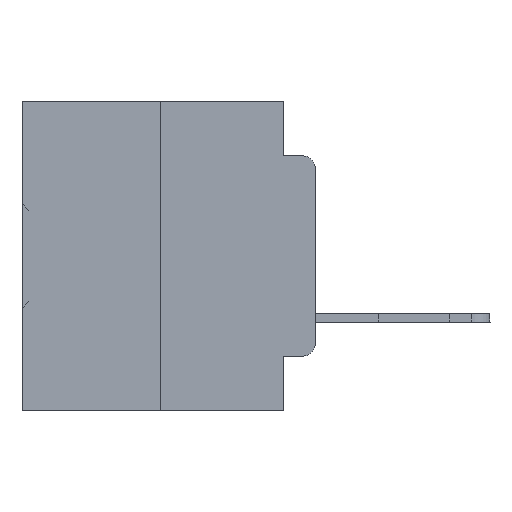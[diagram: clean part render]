
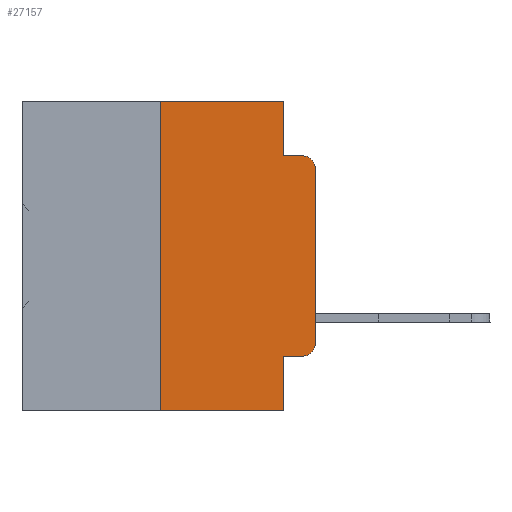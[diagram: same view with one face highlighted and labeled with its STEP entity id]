
A CAD part, left-side view. The second image highlights one B-rep face of the part: STEP entity #27157.
In plain terms, the highlighted planar face has unit normal (-1, 0, 0).
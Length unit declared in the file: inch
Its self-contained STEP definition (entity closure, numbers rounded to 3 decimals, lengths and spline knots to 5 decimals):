
#327 = CARTESIAN_POINT ( 'NONE',  ( 0., 0.25, 0. ) ) ;
#1397 = LINE ( 'NONE', #5929, #7560 ) ;
#1863 = DIRECTION ( 'NONE',  ( 0., -1., 0. ) ) ;
#1883 = CARTESIAN_POINT ( 'NONE',  ( 0., 0.473, 0. ) ) ;
#2228 = DIRECTION ( 'NONE',  ( 0., -1., 0. ) ) ;
#2650 = ORIENTED_EDGE ( 'NONE', *, *, #11590, .T. ) ;
#3807 = CARTESIAN_POINT ( 'NONE',  ( 0., 0., -0.3915 ) ) ;
#3957 = DIRECTION ( 'NONE',  ( 1., 0., 0. ) ) ;
#4090 = EDGE_CURVE ( 'NONE', #22482, #36024, #15081, .T. ) ;
#4218 = DIRECTION ( 'NONE',  ( 0., 0., -1. ) ) ;
#5114 = VECTOR ( 'NONE', #1863, 39.37008 ) ;
#5192 = VECTOR ( 'NONE', #32256, 39.37008 ) ;
#5536 = AXIS2_PLACEMENT_3D ( 'NONE', #11875, #25906, #23444 ) ;
#5929 = CARTESIAN_POINT ( 'NONE',  ( 0., 0.051, 0. ) ) ;
#6291 = LINE ( 'NONE', #33687, #19671 ) ;
#6921 = AXIS2_PLACEMENT_3D ( 'NONE', #27531, #30012, #10509 ) ;
#6992 = ORIENTED_EDGE ( 'NONE', *, *, #33850, .F. ) ;
#7041 = VERTEX_POINT ( 'NONE', #29921 ) ;
#7425 = LINE ( 'NONE', #18552, #5192 ) ;
#7560 = VECTOR ( 'NONE', #31439, 39.37008 ) ;
#8811 = ORIENTED_EDGE ( 'NONE', *, *, #26249, .F. ) ;
#8902 = ORIENTED_EDGE ( 'NONE', *, *, #4090, .T. ) ;
#8966 = AXIS2_PLACEMENT_3D ( 'NONE', #15193, #3957, #4218 ) ;
#9478 = PLANE ( 'NONE',  #8966 ) ;
#10082 = VERTEX_POINT ( 'NONE', #29663 ) ;
#10411 = VERTEX_POINT ( 'NONE', #3807 ) ;
#10509 = DIRECTION ( 'NONE',  ( 0., 0., -1. ) ) ;
#11061 = ORIENTED_EDGE ( 'NONE', *, *, #14763, .T. ) ;
#11104 = CARTESIAN_POINT ( 'NONE',  ( 0., 0.051, -0.0885 ) ) ;
#11590 = EDGE_CURVE ( 'NONE', #36024, #10411, #19796, .T. ) ;
#11759 = CARTESIAN_POINT ( 'NONE',  ( 0., 0.02, -0.4115 ) ) ;
#11875 = CARTESIAN_POINT ( 'NONE',  ( 0., 0.02, -0.1085 ) ) ;
#11906 = VERTEX_POINT ( 'NONE', #15440 ) ;
#12588 = CARTESIAN_POINT ( 'NONE',  ( 0., 0.25, -0.5 ) ) ;
#13746 = ORIENTED_EDGE ( 'NONE', *, *, #13870, .T. ) ;
#13870 = EDGE_CURVE ( 'NONE', #10411, #7041, #6291, .T. ) ;
#14763 = EDGE_CURVE ( 'NONE', #24092, #11906, #30805, .T. ) ;
#15081 = LINE ( 'NONE', #19220, #33770 ) ;
#15193 = CARTESIAN_POINT ( 'NONE',  ( 0., 0.473, 0. ) ) ;
#15335 = VERTEX_POINT ( 'NONE', #11104 ) ;
#15440 = CARTESIAN_POINT ( 'NONE',  ( 0., 0.051, -0.5 ) ) ;
#15716 = CARTESIAN_POINT ( 'NONE',  ( 0., 0.051, 0. ) ) ;
#16206 = DIRECTION ( 'NONE',  ( 0., -1., 0. ) ) ;
#16477 = LINE ( 'NONE', #1883, #19603 ) ;
#16995 = EDGE_CURVE ( 'NONE', #22482, #11906, #1397, .T. ) ;
#18552 = CARTESIAN_POINT ( 'NONE',  ( 0., 0.051, -0.0885 ) ) ;
#19220 = CARTESIAN_POINT ( 'NONE',  ( 0., 0.051, -0.4115 ) ) ;
#19539 = ORIENTED_EDGE ( 'NONE', *, *, #19703, .F. ) ;
#19603 = VECTOR ( 'NONE', #16206, 39.37008 ) ;
#19671 = VECTOR ( 'NONE', #23625, 39.37008 ) ;
#19703 = EDGE_CURVE ( 'NONE', #15335, #10082, #7425, .T. ) ;
#19796 = CIRCLE ( 'NONE', #6921, 0.02 ) ;
#20320 = CARTESIAN_POINT ( 'NONE',  ( 0., 0.051, -0.4115 ) ) ;
#21541 = ORIENTED_EDGE ( 'NONE', *, *, #22009, .T. ) ;
#22009 = EDGE_CURVE ( 'NONE', #7041, #10082, #32736, .T. ) ;
#22166 = VERTEX_POINT ( 'NONE', #23029 ) ;
#22390 = LINE ( 'NONE', #327, #33055 ) ;
#22482 = VERTEX_POINT ( 'NONE', #20320 ) ;
#23029 = CARTESIAN_POINT ( 'NONE',  ( 0., 0.25, 0. ) ) ;
#23444 = DIRECTION ( 'NONE',  ( 0., 0., -1. ) ) ;
#23625 = DIRECTION ( 'NONE',  ( 0., 0., 1. ) ) ;
#23841 = FACE_OUTER_BOUND ( 'NONE', #36456, .T. ) ;
#24092 = VERTEX_POINT ( 'NONE', #12588 ) ;
#24684 = EDGE_CURVE ( 'NONE', #24092, #22166, #22390, .T. ) ;
#25559 = ORIENTED_EDGE ( 'NONE', *, *, #24684, .F. ) ;
#25906 = DIRECTION ( 'NONE',  ( -1., 0., 0. ) ) ;
#26249 = EDGE_CURVE ( 'NONE', #26972, #15335, #30184, .T. ) ;
#26972 = VERTEX_POINT ( 'NONE', #15716 ) ;
#27157 = ADVANCED_FACE ( 'NONE', ( #23841 ), #9478, .F. ) ;
#27531 = CARTESIAN_POINT ( 'NONE',  ( 0., 0.02, -0.3915 ) ) ;
#29663 = CARTESIAN_POINT ( 'NONE',  ( 0., 0.02, -0.0885 ) ) ;
#29921 = CARTESIAN_POINT ( 'NONE',  ( 0., 0., -0.1085 ) ) ;
#30012 = DIRECTION ( 'NONE',  ( -1., 0., 0. ) ) ;
#30184 = LINE ( 'NONE', #31804, #34546 ) ;
#30805 = LINE ( 'NONE', #32811, #5114 ) ;
#31439 = DIRECTION ( 'NONE',  ( 0., 0., -1. ) ) ;
#31804 = CARTESIAN_POINT ( 'NONE',  ( 0., 0.051, 0. ) ) ;
#32256 = DIRECTION ( 'NONE',  ( 0., -1., 0. ) ) ;
#32736 = CIRCLE ( 'NONE', #5536, 0.02 ) ;
#32811 = CARTESIAN_POINT ( 'NONE',  ( 0., 0.473, -0.5 ) ) ;
#33055 = VECTOR ( 'NONE', #34780, 39.37008 ) ;
#33687 = CARTESIAN_POINT ( 'NONE',  ( 0., 0., 0. ) ) ;
#33770 = VECTOR ( 'NONE', #2228, 39.37008 ) ;
#33850 = EDGE_CURVE ( 'NONE', #22166, #26972, #16477, .T. ) ;
#34546 = VECTOR ( 'NONE', #34701, 39.37008 ) ;
#34701 = DIRECTION ( 'NONE',  ( 0., 0., -1. ) ) ;
#34780 = DIRECTION ( 'NONE',  ( 0., 0., 1. ) ) ;
#35754 = ORIENTED_EDGE ( 'NONE', *, *, #16995, .F. ) ;
#36024 = VERTEX_POINT ( 'NONE', #11759 ) ;
#36456 = EDGE_LOOP ( 'NONE', ( #13746, #21541, #19539, #8811, #6992, #25559, #11061, #35754, #8902, #2650 ) ) ;
